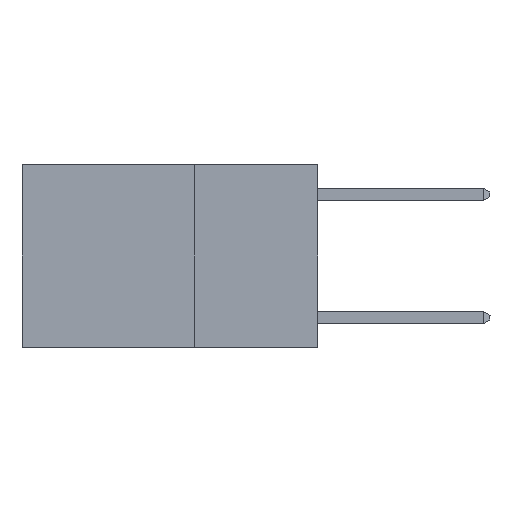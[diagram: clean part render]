
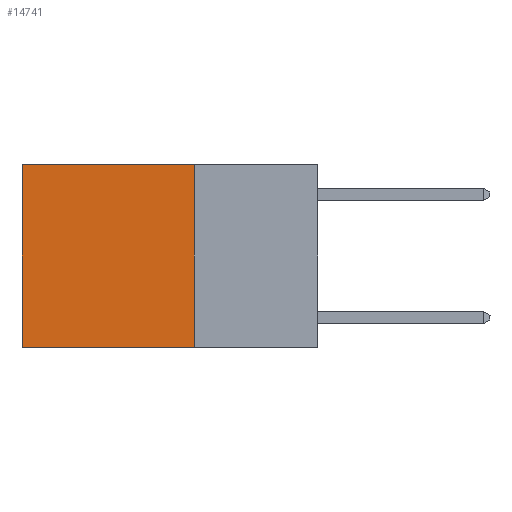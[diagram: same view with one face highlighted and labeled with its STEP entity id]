
A CAD part, left-side view. The second image highlights one B-rep face of the part: STEP entity #14741.
In plain terms, the highlighted planar face has unit normal (-1, 0, 0).
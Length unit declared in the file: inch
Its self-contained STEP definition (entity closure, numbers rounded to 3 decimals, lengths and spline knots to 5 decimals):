
#767 = CARTESIAN_POINT ( 'NONE',  ( 0.2625, 0.25, -0.37 ) ) ;
#2010 = DIRECTION ( 'NONE',  ( 0., 1., 0. ) ) ;
#2402 = EDGE_CURVE ( 'NONE', #6341, #9440, #17980, .T. ) ;
#2526 = CARTESIAN_POINT ( 'NONE',  ( 0.2625, 0.25, 0. ) ) ;
#2930 = ORIENTED_EDGE ( 'NONE', *, *, #5079, .F. ) ;
#3143 = VECTOR ( 'NONE', #14319, 39.37008 ) ;
#3384 = LINE ( 'NONE', #4999, #16873 ) ;
#3729 = CARTESIAN_POINT ( 'NONE',  ( 0.2625, 0.25, 0. ) ) ;
#3925 = VERTEX_POINT ( 'NONE', #767 ) ;
#4257 = DIRECTION ( 'NONE',  ( 0., 0., -1. ) ) ;
#4476 = ORIENTED_EDGE ( 'NONE', *, *, #2402, .T. ) ;
#4999 = CARTESIAN_POINT ( 'NONE',  ( 0.2625, 0.25, -0.37 ) ) ;
#5079 = EDGE_CURVE ( 'NONE', #3925, #8486, #3384, .T. ) ;
#5085 = CARTESIAN_POINT ( 'NONE',  ( 0.2625, 0.6, -0.37 ) ) ;
#5177 = CARTESIAN_POINT ( 'NONE',  ( 0.2625, 0.25, 0. ) ) ;
#6341 = VERTEX_POINT ( 'NONE', #5177 ) ;
#7772 = EDGE_CURVE ( 'NONE', #9440, #8486, #14983, .T. ) ;
#8243 = CARTESIAN_POINT ( 'NONE',  ( 0.2625, 0.6, 0. ) ) ;
#8486 = VERTEX_POINT ( 'NONE', #5085 ) ;
#9064 = VECTOR ( 'NONE', #2010, 39.37008 ) ;
#9440 = VERTEX_POINT ( 'NONE', #15979 ) ;
#9610 = ORIENTED_EDGE ( 'NONE', *, *, #14731, .F. ) ;
#10130 = DIRECTION ( 'NONE',  ( 0., 1., 0. ) ) ;
#11990 = AXIS2_PLACEMENT_3D ( 'NONE', #2526, #14389, #4257 ) ;
#14319 = DIRECTION ( 'NONE',  ( 0., 0., -1. ) ) ;
#14389 = DIRECTION ( 'NONE',  ( 1., 0., 0. ) ) ;
#14731 = EDGE_CURVE ( 'NONE', #6341, #3925, #21000, .T. ) ;
#14741 = ADVANCED_FACE ( 'NONE', ( #19998 ), #20968, .F. ) ;
#14983 = LINE ( 'NONE', #8243, #19408 ) ;
#15979 = CARTESIAN_POINT ( 'NONE',  ( 0.2625, 0.6, 0. ) ) ;
#16012 = CARTESIAN_POINT ( 'NONE',  ( 0.2625, 0.25, 0. ) ) ;
#16873 = VECTOR ( 'NONE', #10130, 39.37008 ) ;
#17197 = EDGE_LOOP ( 'NONE', ( #20156, #2930, #9610, #4476 ) ) ;
#17980 = LINE ( 'NONE', #3729, #9064 ) ;
#19408 = VECTOR ( 'NONE', #19952, 39.37008 ) ;
#19952 = DIRECTION ( 'NONE',  ( 0., 0., -1. ) ) ;
#19998 = FACE_OUTER_BOUND ( 'NONE', #17197, .T. ) ;
#20156 = ORIENTED_EDGE ( 'NONE', *, *, #7772, .T. ) ;
#20968 = PLANE ( 'NONE',  #11990 ) ;
#21000 = LINE ( 'NONE', #16012, #3143 ) ;
